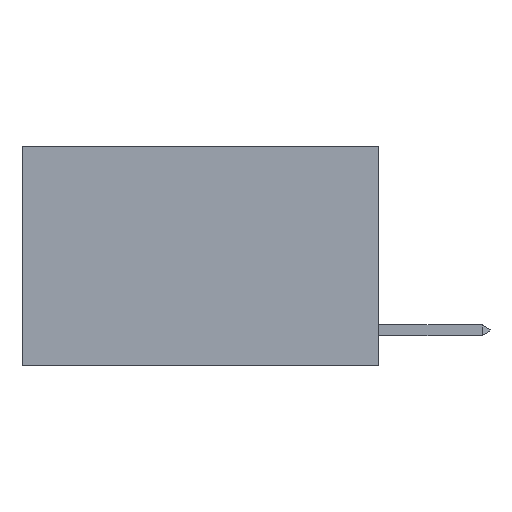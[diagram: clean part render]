
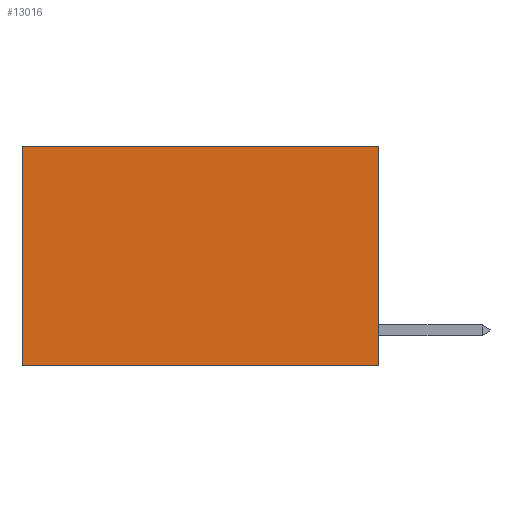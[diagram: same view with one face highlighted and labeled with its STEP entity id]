
A CAD part, left-side view. The second image highlights one B-rep face of the part: STEP entity #13016.
In plain terms, the highlighted planar face has unit normal (-1, 0, 0).
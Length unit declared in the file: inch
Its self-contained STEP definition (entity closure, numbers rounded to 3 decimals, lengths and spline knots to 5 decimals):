
#429 = PLANE ( 'NONE',  #1676 ) ;
#935 = VECTOR ( 'NONE', #14400, 39.37008 ) ;
#997 = ORIENTED_EDGE ( 'NONE', *, *, #18141, .F. ) ;
#1356 = EDGE_CURVE ( 'NONE', #11075, #1898, #9824, .T. ) ;
#1676 = AXIS2_PLACEMENT_3D ( 'NONE', #8233, #6618, #14642 ) ;
#1898 = VERTEX_POINT ( 'NONE', #8830 ) ;
#2007 = CARTESIAN_POINT ( 'NONE',  ( 0.2625, 0.6, 0. ) ) ;
#2244 = CARTESIAN_POINT ( 'NONE',  ( 0.2625, 0., -0.37 ) ) ;
#2675 = CARTESIAN_POINT ( 'NONE',  ( 0.2625, 0.6, 0. ) ) ;
#2740 = CARTESIAN_POINT ( 'NONE',  ( 0.2625, 0., 0. ) ) ;
#3242 = VERTEX_POINT ( 'NONE', #7384 ) ;
#4504 = DIRECTION ( 'NONE',  ( 0., 1., 0. ) ) ;
#4632 = ORIENTED_EDGE ( 'NONE', *, *, #12330, .T. ) ;
#6144 = EDGE_CURVE ( 'NONE', #13000, #1898, #14492, .T. ) ;
#6618 = DIRECTION ( 'NONE',  ( 1., 0., 0. ) ) ;
#6770 = CARTESIAN_POINT ( 'NONE',  ( 0.2625, 0., -0.37 ) ) ;
#7221 = DIRECTION ( 'NONE',  ( 0., 0., -1. ) ) ;
#7384 = CARTESIAN_POINT ( 'NONE',  ( 0.2625, 0., 0. ) ) ;
#8233 = CARTESIAN_POINT ( 'NONE',  ( 0.2625, 0., 0. ) ) ;
#8279 = ORIENTED_EDGE ( 'NONE', *, *, #1356, .T. ) ;
#8830 = CARTESIAN_POINT ( 'NONE',  ( 0.2625, 0.6, -0.37 ) ) ;
#9824 = LINE ( 'NONE', #2007, #935 ) ;
#11075 = VERTEX_POINT ( 'NONE', #2675 ) ;
#11500 = VECTOR ( 'NONE', #12984, 39.37008 ) ;
#12113 = EDGE_LOOP ( 'NONE', ( #8279, #19178, #997, #4632 ) ) ;
#12231 = CARTESIAN_POINT ( 'NONE',  ( 0.2625, 0., 0. ) ) ;
#12330 = EDGE_CURVE ( 'NONE', #3242, #11075, #19974, .T. ) ;
#12984 = DIRECTION ( 'NONE',  ( 0., 1., 0. ) ) ;
#13000 = VERTEX_POINT ( 'NONE', #2244 ) ;
#13016 = ADVANCED_FACE ( 'NONE', ( #14345 ), #429, .F. ) ;
#14314 = VECTOR ( 'NONE', #4504, 39.37008 ) ;
#14345 = FACE_OUTER_BOUND ( 'NONE', #12113, .T. ) ;
#14400 = DIRECTION ( 'NONE',  ( 0., 0., -1. ) ) ;
#14492 = LINE ( 'NONE', #6770, #11500 ) ;
#14642 = DIRECTION ( 'NONE',  ( 0., 0., -1. ) ) ;
#18032 = VECTOR ( 'NONE', #7221, 39.37008 ) ;
#18141 = EDGE_CURVE ( 'NONE', #3242, #13000, #19743, .T. ) ;
#19178 = ORIENTED_EDGE ( 'NONE', *, *, #6144, .F. ) ;
#19743 = LINE ( 'NONE', #2740, #18032 ) ;
#19974 = LINE ( 'NONE', #12231, #14314 ) ;
